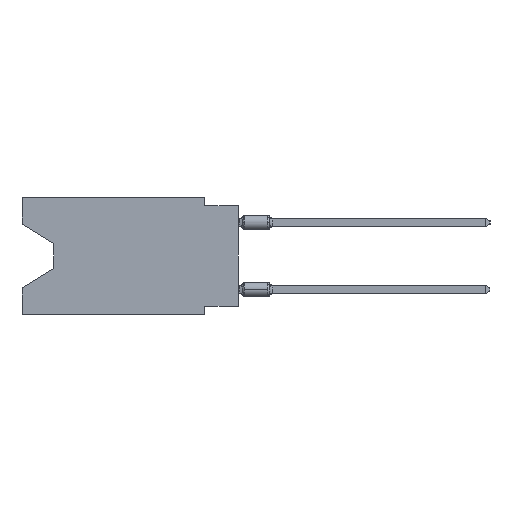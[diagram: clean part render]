
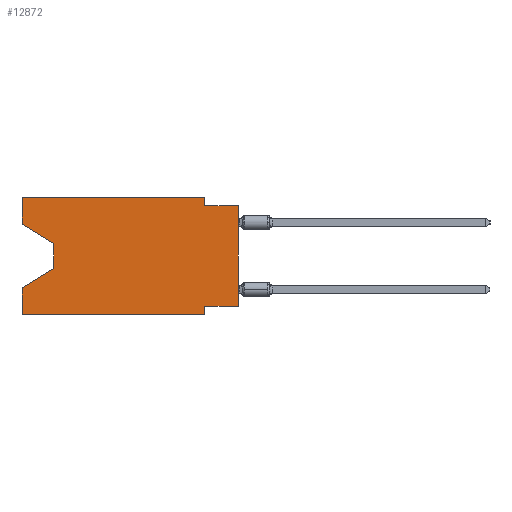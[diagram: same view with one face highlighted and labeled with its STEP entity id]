
A CAD part, left-side view. The second image highlights one B-rep face of the part: STEP entity #12872.
In plain terms, the highlighted planar face has unit normal (-1, 0, 0).
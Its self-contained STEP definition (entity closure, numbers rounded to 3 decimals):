
#679 = EDGE_CURVE ( 'NONE', #11817, #37220, #2805, .T. ) ;
#2082 = DIRECTION ( 'NONE',  ( 0., 0.855, -0.519 ) ) ;
#2282 = DIRECTION ( 'NONE',  ( 0., -1., 0. ) ) ;
#2428 = VECTOR ( 'NONE', #2082, 1000. ) ;
#2453 = CARTESIAN_POINT ( 'NONE',  ( 0., 16.383, 0. ) ) ;
#2712 = ORIENTED_EDGE ( 'NONE', *, *, #37756, .T. ) ;
#2733 = EDGE_CURVE ( 'NONE', #38810, #3163, #31999, .T. ) ;
#2805 = LINE ( 'NONE', #42074, #20120 ) ;
#3163 = VERTEX_POINT ( 'NONE', #21947 ) ;
#3478 = LINE ( 'NONE', #14103, #25816 ) ;
#3547 = VERTEX_POINT ( 'NONE', #22542 ) ;
#3992 = CARTESIAN_POINT ( 'NONE',  ( 0., 2.54, -8.255 ) ) ;
#4174 = EDGE_CURVE ( 'NONE', #10482, #10406, #29539, .T. ) ;
#5324 = VECTOR ( 'NONE', #12853, 1000. ) ;
#5733 = CARTESIAN_POINT ( 'NONE',  ( 0., 0., -0.635 ) ) ;
#7684 = ORIENTED_EDGE ( 'NONE', *, *, #9453, .F. ) ;
#7946 = ORIENTED_EDGE ( 'NONE', *, *, #679, .T. ) ;
#8130 = CARTESIAN_POINT ( 'NONE',  ( 0., 13.97, -5.385 ) ) ;
#8325 = ORIENTED_EDGE ( 'NONE', *, *, #2733, .F. ) ;
#8562 = EDGE_LOOP ( 'NONE', ( #9533, #7946, #10425, #21140, #2712, #8325, #10469, #23257, #7684, #42730, #36324, #18457 ) ) ;
#9283 = CARTESIAN_POINT ( 'NONE',  ( 0., 13.97, -3.505 ) ) ;
#9453 = EDGE_CURVE ( 'NONE', #27592, #12513, #18754, .T. ) ;
#9533 = ORIENTED_EDGE ( 'NONE', *, *, #19030, .T. ) ;
#9793 = LINE ( 'NONE', #12623, #26587 ) ;
#9883 = VERTEX_POINT ( 'NONE', #19554 ) ;
#9902 = EDGE_CURVE ( 'NONE', #9883, #12513, #32822, .T. ) ;
#9961 = CARTESIAN_POINT ( 'NONE',  ( 0., 16.383, 0. ) ) ;
#10382 = PLANE ( 'NONE',  #31312 ) ;
#10406 = VERTEX_POINT ( 'NONE', #30720 ) ;
#10425 = ORIENTED_EDGE ( 'NONE', *, *, #14890, .T. ) ;
#10469 = ORIENTED_EDGE ( 'NONE', *, *, #39827, .F. ) ;
#10482 = VERTEX_POINT ( 'NONE', #20309 ) ;
#11817 = VERTEX_POINT ( 'NONE', #9283 ) ;
#12347 = DIRECTION ( 'NONE',  ( 0., 0., -1. ) ) ;
#12434 = DIRECTION ( 'NONE',  ( 0., 0., 1. ) ) ;
#12513 = VERTEX_POINT ( 'NONE', #19070 ) ;
#12623 = CARTESIAN_POINT ( 'NONE',  ( 0., 16.383, -8.89 ) ) ;
#12853 = DIRECTION ( 'NONE',  ( 0., 0., 1. ) ) ;
#12872 = ADVANCED_FACE ( 'NONE', ( #26885 ), #10382, .F. ) ;
#12907 = CARTESIAN_POINT ( 'NONE',  ( 0., 2.54, -8.89 ) ) ;
#13701 = CARTESIAN_POINT ( 'NONE',  ( 0., 16.383, -2.038 ) ) ;
#14103 = CARTESIAN_POINT ( 'NONE',  ( 0., 2.54, 0. ) ) ;
#14238 = VECTOR ( 'NONE', #25980, 1000. ) ;
#14890 = EDGE_CURVE ( 'NONE', #37220, #10406, #25051, .T. ) ;
#15658 = DIRECTION ( 'NONE',  ( 0., -1., 0. ) ) ;
#15717 = DIRECTION ( 'NONE',  ( 0., 0., -1. ) ) ;
#16392 = CARTESIAN_POINT ( 'NONE',  ( 0., 16.383, 0. ) ) ;
#16693 = CARTESIAN_POINT ( 'NONE',  ( 0., 2.54, -0.635 ) ) ;
#17364 = LINE ( 'NONE', #13701, #18722 ) ;
#18389 = CARTESIAN_POINT ( 'NONE',  ( 0., 16.383, -2.038 ) ) ;
#18457 = ORIENTED_EDGE ( 'NONE', *, *, #30358, .F. ) ;
#18722 = VECTOR ( 'NONE', #20174, 1000. ) ;
#18754 = LINE ( 'NONE', #5733, #25379 ) ;
#19030 = EDGE_CURVE ( 'NONE', #24828, #11817, #17364, .T. ) ;
#19070 = CARTESIAN_POINT ( 'NONE',  ( 0., 0., -0.635 ) ) ;
#19554 = CARTESIAN_POINT ( 'NONE',  ( 0., 0., -8.255 ) ) ;
#19599 = EDGE_CURVE ( 'NONE', #35507, #3547, #30557, .T. ) ;
#20120 = VECTOR ( 'NONE', #12347, 1000. ) ;
#20174 = DIRECTION ( 'NONE',  ( 0., -0.855, -0.519 ) ) ;
#20309 = CARTESIAN_POINT ( 'NONE',  ( 0., 16.383, -8.89 ) ) ;
#20598 = DIRECTION ( 'NONE',  ( 0., 0., -1. ) ) ;
#20730 = VECTOR ( 'NONE', #12434, 1000. ) ;
#21140 = ORIENTED_EDGE ( 'NONE', *, *, #4174, .F. ) ;
#21947 = CARTESIAN_POINT ( 'NONE',  ( 0., 2.54, -8.89 ) ) ;
#21973 = LINE ( 'NONE', #2453, #20730 ) ;
#21994 = EDGE_CURVE ( 'NONE', #3547, #27592, #3478, .T. ) ;
#22501 = CARTESIAN_POINT ( 'NONE',  ( 0., 0., -8.255 ) ) ;
#22542 = CARTESIAN_POINT ( 'NONE',  ( 0., 2.54, 0. ) ) ;
#22573 = DIRECTION ( 'NONE',  ( 0., 0., 1. ) ) ;
#23257 = ORIENTED_EDGE ( 'NONE', *, *, #9902, .T. ) ;
#24654 = CARTESIAN_POINT ( 'NONE',  ( 0., 16.383, 0. ) ) ;
#24828 = VERTEX_POINT ( 'NONE', #18389 ) ;
#25051 = LINE ( 'NONE', #31802, #2428 ) ;
#25379 = VECTOR ( 'NONE', #2282, 1000. ) ;
#25816 = VECTOR ( 'NONE', #20598, 1000. ) ;
#25980 = DIRECTION ( 'NONE',  ( 0., 1., 0. ) ) ;
#26452 = VECTOR ( 'NONE', #30976, 1000. ) ;
#26587 = VECTOR ( 'NONE', #15658, 1000. ) ;
#26885 = FACE_OUTER_BOUND ( 'NONE', #8562, .T. ) ;
#27592 = VERTEX_POINT ( 'NONE', #16693 ) ;
#28899 = VECTOR ( 'NONE', #15717, 1000. ) ;
#28997 = VECTOR ( 'NONE', #22573, 1000. ) ;
#29025 = LINE ( 'NONE', #22501, #14238 ) ;
#29539 = LINE ( 'NONE', #42774, #28997 ) ;
#30358 = EDGE_CURVE ( 'NONE', #24828, #35507, #21973, .T. ) ;
#30557 = LINE ( 'NONE', #24654, #26452 ) ;
#30720 = CARTESIAN_POINT ( 'NONE',  ( 0., 16.383, -6.852 ) ) ;
#30976 = DIRECTION ( 'NONE',  ( 0., -1., 0. ) ) ;
#31312 = AXIS2_PLACEMENT_3D ( 'NONE', #9961, #39895, #40534 ) ;
#31802 = CARTESIAN_POINT ( 'NONE',  ( 0., 13.97, -5.385 ) ) ;
#31999 = LINE ( 'NONE', #12907, #28899 ) ;
#32822 = LINE ( 'NONE', #42578, #5324 ) ;
#35507 = VERTEX_POINT ( 'NONE', #16392 ) ;
#36324 = ORIENTED_EDGE ( 'NONE', *, *, #19599, .F. ) ;
#37220 = VERTEX_POINT ( 'NONE', #8130 ) ;
#37756 = EDGE_CURVE ( 'NONE', #10482, #3163, #9793, .T. ) ;
#38810 = VERTEX_POINT ( 'NONE', #3992 ) ;
#39827 = EDGE_CURVE ( 'NONE', #9883, #38810, #29025, .T. ) ;
#39895 = DIRECTION ( 'NONE',  ( 1., 0., 0. ) ) ;
#40534 = DIRECTION ( 'NONE',  ( 0., 0., -1. ) ) ;
#42074 = CARTESIAN_POINT ( 'NONE',  ( 0., 13.97, -3.505 ) ) ;
#42578 = CARTESIAN_POINT ( 'NONE',  ( 0., 0., 0. ) ) ;
#42730 = ORIENTED_EDGE ( 'NONE', *, *, #21994, .F. ) ;
#42774 = CARTESIAN_POINT ( 'NONE',  ( 0., 16.383, 0. ) ) ;
